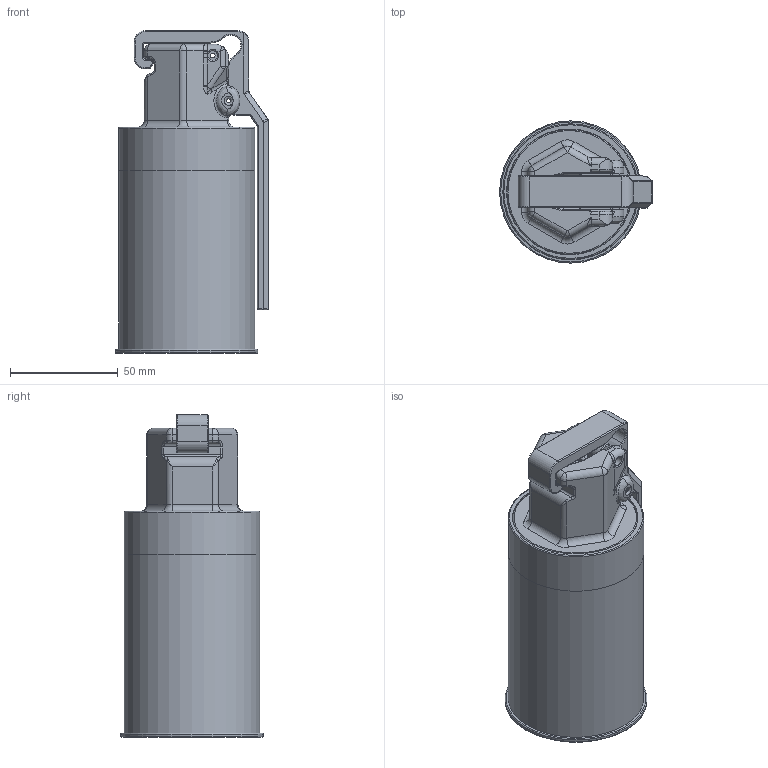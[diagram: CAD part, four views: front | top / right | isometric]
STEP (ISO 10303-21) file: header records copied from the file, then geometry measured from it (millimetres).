
FILE_DESCRIPTION(/* description */ (''),/* implementation_level */ '2;1');
FILE_NAME(/* name */ 'M18.stp',/* time_stamp */ '2019-12-09T18:02:49+02:00',/* author */ (''),/* organization */ (''),/* preprocessor_version */ 'ST-DEVELOPER v15.2',/* originating_system */ 'Autodesk Translator Framework v2.0.0.5431',/* authorisation */ '');
FILE_SCHEMA (('AUTOMOTIVE_DESIGN { 1 0 10303 214 3 1 1 }'));
Length unit declared in the file: centimetre
Products named in the file (1): SMOKE GRENADE M18 V6
Bounding box: 70.91 x 66 x 149.85 mm (x, y, z)
Volume: 137546.4 mm3; surface area: 72504.6 mm2
Topology: 5 solids, 5 shells, 391 faces, 927 edges, 534 vertices
Faces by surface type: cylinder 162, plane 84, bspline 80, torus 56, sphere 6, cone 3
Full cylindrical faces by diameter (mm): 0.2 x1, 2 x1, 2.1 x2, 2.15 x2, 2.57 x1, 3 x1, 4.51 x2, 15 x1, 53.199 x1, 56.502 x1, 57 x1, 58 x1, 58.4 x1, 63 x1, 63.018 x1, 66 x1
Entity records: 13477 total; most frequent: CARTESIAN_POINT 4795, DIRECTION 1840, ORIENTED_EDGE 1758, EDGE_CURVE 879, AXIS2_PLACEMENT_3D 757, VERTEX_POINT 529, EDGE_LOOP 442, ADVANCED_FACE 391
